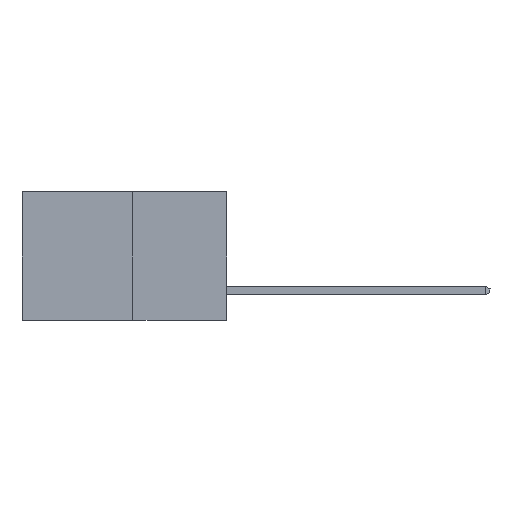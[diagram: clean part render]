
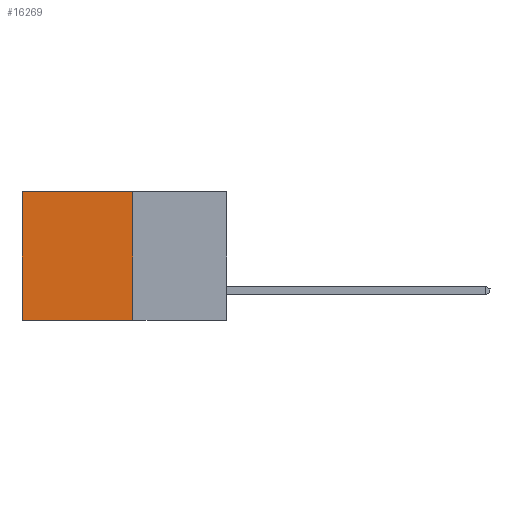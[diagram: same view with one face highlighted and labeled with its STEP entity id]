
A CAD part, left-side view. The second image highlights one B-rep face of the part: STEP entity #16269.
In plain terms, the highlighted planar face has unit normal (-1, 0, 0).
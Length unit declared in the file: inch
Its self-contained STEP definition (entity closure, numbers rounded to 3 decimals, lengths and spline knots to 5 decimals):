
#299 = EDGE_LOOP ( 'NONE', ( #10712, #5343, #10061, #8070 ) ) ;
#1168 = VERTEX_POINT ( 'NONE', #15996 ) ;
#1311 = CARTESIAN_POINT ( 'NONE',  ( 0.277, 0.27, -0.37 ) ) ;
#1483 = CARTESIAN_POINT ( 'NONE',  ( 0.277, 0.27, -0.37 ) ) ;
#1710 = EDGE_CURVE ( 'NONE', #1168, #9609, #13462, .T. ) ;
#3966 = CARTESIAN_POINT ( 'NONE',  ( 0.277, 0.27, -0.37 ) ) ;
#4348 = DIRECTION ( 'NONE',  ( 0., 0., -1. ) ) ;
#4725 = DIRECTION ( 'NONE',  ( 0., 0., -1. ) ) ;
#4818 = VECTOR ( 'NONE', #4725, 39.37008 ) ;
#4924 = CARTESIAN_POINT ( 'NONE',  ( 0.277, 0.59, 0. ) ) ;
#5343 = ORIENTED_EDGE ( 'NONE', *, *, #5750, .F. ) ;
#5373 = FACE_OUTER_BOUND ( 'NONE', #299, .T. ) ;
#5750 = EDGE_CURVE ( 'NONE', #6390, #14966, #17300, .T. ) ;
#5859 = VECTOR ( 'NONE', #17968, 39.37008 ) ;
#6128 = PLANE ( 'NONE',  #10293 ) ;
#6390 = VERTEX_POINT ( 'NONE', #1311 ) ;
#6714 = EDGE_CURVE ( 'NONE', #9609, #14966, #12433, .T. ) ;
#8070 = ORIENTED_EDGE ( 'NONE', *, *, #1710, .T. ) ;
#8371 = CARTESIAN_POINT ( 'NONE',  ( 0.277, 0.27, 0. ) ) ;
#9108 = CARTESIAN_POINT ( 'NONE',  ( 0.277, 0.27, -0.37 ) ) ;
#9190 = DIRECTION ( 'NONE',  ( 0., 1., 0. ) ) ;
#9609 = VERTEX_POINT ( 'NONE', #4924 ) ;
#10061 = ORIENTED_EDGE ( 'NONE', *, *, #14940, .F. ) ;
#10293 = AXIS2_PLACEMENT_3D ( 'NONE', #1483, #12902, #4348 ) ;
#10712 = ORIENTED_EDGE ( 'NONE', *, *, #6714, .T. ) ;
#12433 = LINE ( 'NONE', #14268, #4818 ) ;
#12902 = DIRECTION ( 'NONE',  ( 1., 0., 0. ) ) ;
#13462 = LINE ( 'NONE', #8371, #5859 ) ;
#13476 = LINE ( 'NONE', #3966, #16800 ) ;
#13995 = DIRECTION ( 'NONE',  ( 0., 0., -1. ) ) ;
#14061 = CARTESIAN_POINT ( 'NONE',  ( 0.277, 0.59, -0.37 ) ) ;
#14268 = CARTESIAN_POINT ( 'NONE',  ( 0.277, 0.59, -0.37 ) ) ;
#14940 = EDGE_CURVE ( 'NONE', #1168, #6390, #13476, .T. ) ;
#14966 = VERTEX_POINT ( 'NONE', #14061 ) ;
#15996 = CARTESIAN_POINT ( 'NONE',  ( 0.277, 0.27, 0. ) ) ;
#16269 = ADVANCED_FACE ( 'NONE', ( #5373 ), #6128, .F. ) ;
#16800 = VECTOR ( 'NONE', #13995, 39.37008 ) ;
#17300 = LINE ( 'NONE', #9108, #18171 ) ;
#17968 = DIRECTION ( 'NONE',  ( 0., 1., 0. ) ) ;
#18171 = VECTOR ( 'NONE', #9190, 39.37008 ) ;
